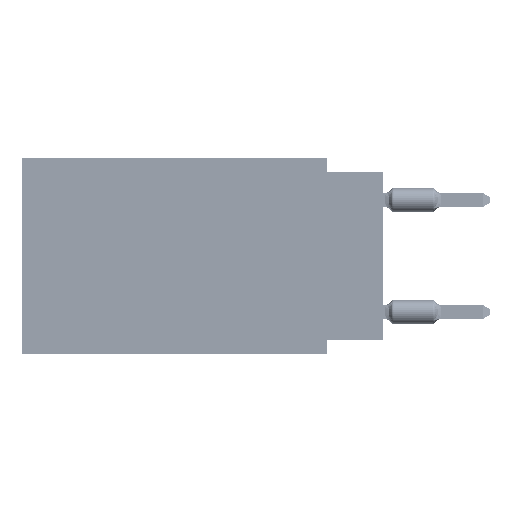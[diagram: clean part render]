
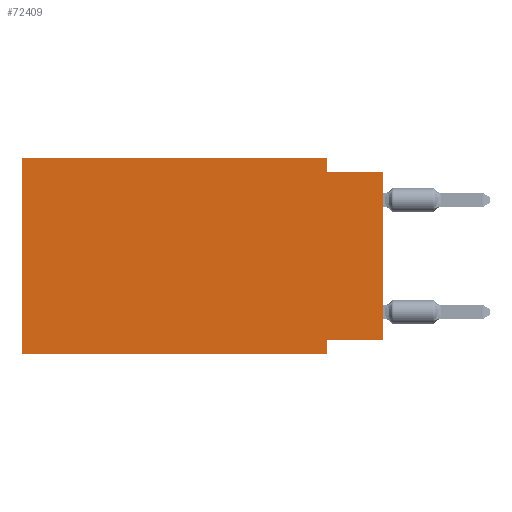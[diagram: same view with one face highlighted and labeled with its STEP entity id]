
A CAD part, left-side view. The second image highlights one B-rep face of the part: STEP entity #72409.
In plain terms, the highlighted planar face has unit normal (-1, 0, 0).
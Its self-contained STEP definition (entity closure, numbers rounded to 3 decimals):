
#1449 = VECTOR ( 'NONE', #34129, 1000. ) ;
#1611 = VECTOR ( 'NONE', #18089, 1000. ) ;
#4409 = CARTESIAN_POINT ( 'NONE',  ( 0., 16.383, -8.89 ) ) ;
#4690 = VECTOR ( 'NONE', #26472, 1000. ) ;
#5110 = CARTESIAN_POINT ( 'NONE',  ( 0., 16.383, 0. ) ) ;
#6564 = VERTEX_POINT ( 'NONE', #11911 ) ;
#7291 = EDGE_CURVE ( 'NONE', #30909, #32531, #24022, .T. ) ;
#8030 = CARTESIAN_POINT ( 'NONE',  ( 0., 2.54, -8.89 ) ) ;
#8970 = LINE ( 'NONE', #54760, #57477 ) ;
#9084 = CARTESIAN_POINT ( 'NONE',  ( 0., 0., -8.255 ) ) ;
#9919 = DIRECTION ( 'NONE',  ( 0., 1., 0. ) ) ;
#10772 = DIRECTION ( 'NONE',  ( 0., 0., 1. ) ) ;
#11911 = CARTESIAN_POINT ( 'NONE',  ( 0., 2.54, -8.89 ) ) ;
#11974 = EDGE_CURVE ( 'NONE', #30909, #49329, #42031, .T. ) ;
#16641 = DIRECTION ( 'NONE',  ( 0., 0., 1. ) ) ;
#17231 = DIRECTION ( 'NONE',  ( 0., -1., 0. ) ) ;
#18089 = DIRECTION ( 'NONE',  ( 0., -1., 0. ) ) ;
#19072 = VECTOR ( 'NONE', #79257, 1000. ) ;
#21881 = ORIENTED_EDGE ( 'NONE', *, *, #27416, .F. ) ;
#21935 = CARTESIAN_POINT ( 'NONE',  ( 0., 2.54, 0. ) ) ;
#22694 = ORIENTED_EDGE ( 'NONE', *, *, #31679, .F. ) ;
#24022 = LINE ( 'NONE', #82697, #38334 ) ;
#24672 = EDGE_CURVE ( 'NONE', #75866, #32531, #38179, .T. ) ;
#25391 = ORIENTED_EDGE ( 'NONE', *, *, #11974, .F. ) ;
#26472 = DIRECTION ( 'NONE',  ( 0., 0., -1. ) ) ;
#26671 = EDGE_CURVE ( 'NONE', #43798, #6564, #70726, .T. ) ;
#27071 = ORIENTED_EDGE ( 'NONE', *, *, #26671, .T. ) ;
#27416 = EDGE_CURVE ( 'NONE', #43798, #62472, #8970, .T. ) ;
#27457 = LINE ( 'NONE', #41135, #19072 ) ;
#30896 = CARTESIAN_POINT ( 'NONE',  ( 0., 0., -0.635 ) ) ;
#30909 = VERTEX_POINT ( 'NONE', #69812 ) ;
#31215 = FACE_OUTER_BOUND ( 'NONE', #31534, .T. ) ;
#31389 = CARTESIAN_POINT ( 'NONE',  ( 0., 2.54, -8.255 ) ) ;
#31534 = EDGE_LOOP ( 'NONE', ( #35016, #61757, #22694, #54316, #21881, #27071, #56731, #25391 ) ) ;
#31679 = EDGE_CURVE ( 'NONE', #59824, #75866, #50561, .T. ) ;
#32503 = CARTESIAN_POINT ( 'NONE',  ( 0., 16.383, 0. ) ) ;
#32531 = VERTEX_POINT ( 'NONE', #66058 ) ;
#32797 = CARTESIAN_POINT ( 'NONE',  ( 0., 16.383, -8.89 ) ) ;
#34129 = DIRECTION ( 'NONE',  ( 0., 0., -1. ) ) ;
#35016 = ORIENTED_EDGE ( 'NONE', *, *, #7291, .T. ) ;
#37722 = CARTESIAN_POINT ( 'NONE',  ( 0., 2.54, 0. ) ) ;
#38179 = LINE ( 'NONE', #30896, #43405 ) ;
#38334 = VECTOR ( 'NONE', #10772, 1000. ) ;
#40094 = EDGE_CURVE ( 'NONE', #49329, #6564, #66650, .T. ) ;
#41135 = CARTESIAN_POINT ( 'NONE',  ( 0., 16.383, 0. ) ) ;
#42031 = LINE ( 'NONE', #9084, #68965 ) ;
#43405 = VECTOR ( 'NONE', #17231, 1000. ) ;
#43798 = VERTEX_POINT ( 'NONE', #32797 ) ;
#49329 = VERTEX_POINT ( 'NONE', #31389 ) ;
#50561 = LINE ( 'NONE', #37722, #4690 ) ;
#54316 = ORIENTED_EDGE ( 'NONE', *, *, #73225, .F. ) ;
#54760 = CARTESIAN_POINT ( 'NONE',  ( 0., 16.383, 0. ) ) ;
#56731 = ORIENTED_EDGE ( 'NONE', *, *, #40094, .F. ) ;
#57352 = CARTESIAN_POINT ( 'NONE',  ( 0., 2.54, -0.635 ) ) ;
#57477 = VECTOR ( 'NONE', #16641, 1000. ) ;
#59824 = VERTEX_POINT ( 'NONE', #21935 ) ;
#61757 = ORIENTED_EDGE ( 'NONE', *, *, #24672, .F. ) ;
#62472 = VERTEX_POINT ( 'NONE', #32503 ) ;
#64161 = PLANE ( 'NONE',  #66864 ) ;
#66058 = CARTESIAN_POINT ( 'NONE',  ( 0., 0., -0.635 ) ) ;
#66650 = LINE ( 'NONE', #8030, #1449 ) ;
#66864 = AXIS2_PLACEMENT_3D ( 'NONE', #5110, #77882, #71018 ) ;
#68965 = VECTOR ( 'NONE', #9919, 1000. ) ;
#69812 = CARTESIAN_POINT ( 'NONE',  ( 0., 0., -8.255 ) ) ;
#70726 = LINE ( 'NONE', #4409, #1611 ) ;
#71018 = DIRECTION ( 'NONE',  ( 0., 0., -1. ) ) ;
#72409 = ADVANCED_FACE ( 'NONE', ( #31215 ), #64161, .F. ) ;
#73225 = EDGE_CURVE ( 'NONE', #62472, #59824, #27457, .T. ) ;
#75866 = VERTEX_POINT ( 'NONE', #57352 ) ;
#77882 = DIRECTION ( 'NONE',  ( 1., 0., 0. ) ) ;
#79257 = DIRECTION ( 'NONE',  ( 0., -1., 0. ) ) ;
#82697 = CARTESIAN_POINT ( 'NONE',  ( 0., 0., 0. ) ) ;
